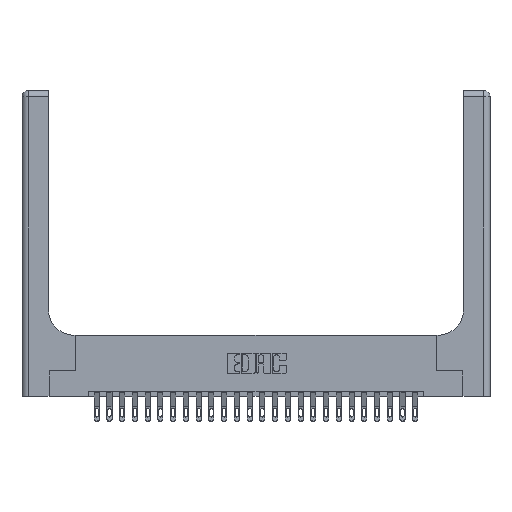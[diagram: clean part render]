
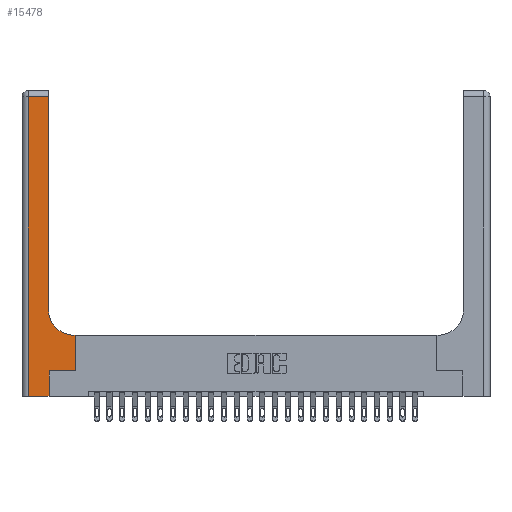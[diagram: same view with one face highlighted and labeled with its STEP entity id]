
A CAD part, top view. The second image highlights one B-rep face of the part: STEP entity #15478.
In plain terms, the highlighted planar face has unit normal (0, 0, 1).
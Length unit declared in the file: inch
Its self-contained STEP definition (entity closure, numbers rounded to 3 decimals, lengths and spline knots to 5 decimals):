
#1014 = CARTESIAN_POINT ( 'NONE',  ( 0.26, 0.85, 0.37 ) ) ;
#1389 = EDGE_CURVE ( 'NONE', #7371, #19761, #3954, .T. ) ;
#1465 = LINE ( 'NONE', #8981, #24023 ) ;
#1598 = ORIENTED_EDGE ( 'NONE', *, *, #18010, .T. ) ;
#1898 = EDGE_CURVE ( 'NONE', #4149, #11383, #24601, .T. ) ;
#1945 = LINE ( 'NONE', #6008, #16752 ) ;
#2330 = DIRECTION ( 'NONE',  ( 0., 1., 0. ) ) ;
#3013 = VECTOR ( 'NONE', #18596, 39.37008 ) ;
#3954 = CIRCLE ( 'NONE', #10452, 0.25 ) ;
#4149 = VERTEX_POINT ( 'NONE', #20204 ) ;
#4366 = DIRECTION ( 'NONE',  ( 0., 1., 0. ) ) ;
#4410 = VERTEX_POINT ( 'NONE', #11803 ) ;
#4549 = EDGE_LOOP ( 'NONE', ( #18722, #13745, #19263, #1598, #19499, #21792, #6718, #7309, #8735 ) ) ;
#5211 = CARTESIAN_POINT ( 'NONE',  ( 0., 2.94, 0.37 ) ) ;
#6008 = CARTESIAN_POINT ( 'NONE',  ( 0., 0., 0.37 ) ) ;
#6191 = DIRECTION ( 'NONE',  ( -1., 0., 0. ) ) ;
#6286 = CARTESIAN_POINT ( 'NONE',  ( 0.265, 0., 0.37 ) ) ;
#6718 = ORIENTED_EDGE ( 'NONE', *, *, #10161, .T. ) ;
#7309 = ORIENTED_EDGE ( 'NONE', *, *, #24909, .T. ) ;
#7371 = VERTEX_POINT ( 'NONE', #11043 ) ;
#7936 = LINE ( 'NONE', #15918, #16631 ) ;
#8138 = CARTESIAN_POINT ( 'NONE',  ( 0.26, 0.6, 0.37 ) ) ;
#8153 = CARTESIAN_POINT ( 'NONE',  ( 0.06, 2.94, 0.37 ) ) ;
#8735 = ORIENTED_EDGE ( 'NONE', *, *, #1389, .T. ) ;
#8981 = CARTESIAN_POINT ( 'NONE',  ( 0.26, 3., 0.37 ) ) ;
#9697 = DIRECTION ( 'NONE',  ( 1., 0., 0. ) ) ;
#9804 = AXIS2_PLACEMENT_3D ( 'NONE', #15721, #9871, #6191 ) ;
#9871 = DIRECTION ( 'NONE',  ( 0., 0., -1. ) ) ;
#10161 = EDGE_CURVE ( 'NONE', #11383, #4410, #7936, .T. ) ;
#10452 = AXIS2_PLACEMENT_3D ( 'NONE', #15229, #15479, #13464 ) ;
#11038 = CARTESIAN_POINT ( 'NONE',  ( 0.06, 0., 0.37 ) ) ;
#11043 = CARTESIAN_POINT ( 'NONE',  ( 0.51, 0.6, 0.37 ) ) ;
#11187 = VECTOR ( 'NONE', #25009, 39.37008 ) ;
#11383 = VERTEX_POINT ( 'NONE', #19030 ) ;
#11803 = CARTESIAN_POINT ( 'NONE',  ( 0.528, 0.6, 0.37 ) ) ;
#12971 = DIRECTION ( 'NONE',  ( -1., 0., 0. ) ) ;
#13177 = CARTESIAN_POINT ( 'NONE',  ( 0.265, 0.25, 0.37 ) ) ;
#13186 = EDGE_CURVE ( 'NONE', #17168, #4149, #23682, .T. ) ;
#13464 = DIRECTION ( 'NONE',  ( 1., 0., 0. ) ) ;
#13709 = LINE ( 'NONE', #21306, #14698 ) ;
#13745 = ORIENTED_EDGE ( 'NONE', *, *, #19863, .T. ) ;
#14698 = VECTOR ( 'NONE', #19912, 39.37008 ) ;
#15229 = CARTESIAN_POINT ( 'NONE',  ( 0.51, 0.85, 0.37 ) ) ;
#15267 = VERTEX_POINT ( 'NONE', #11038 ) ;
#15450 = EDGE_CURVE ( 'NONE', #21460, #15267, #13709, .T. ) ;
#15478 = ADVANCED_FACE ( 'NONE', ( #19655 ), #19789, .F. ) ;
#15479 = DIRECTION ( 'NONE',  ( 0., 0., -1. ) ) ;
#15721 = CARTESIAN_POINT ( 'NONE',  ( 0., 3., 0.37 ) ) ;
#15857 = EDGE_CURVE ( 'NONE', #19761, #17835, #1465, .T. ) ;
#15918 = CARTESIAN_POINT ( 'NONE',  ( 0.528, 0.25, 0.37 ) ) ;
#16631 = VECTOR ( 'NONE', #2330, 39.37008 ) ;
#16752 = VECTOR ( 'NONE', #9697, 39.37008 ) ;
#17168 = VERTEX_POINT ( 'NONE', #20784 ) ;
#17288 = LINE ( 'NONE', #8138, #11187 ) ;
#17835 = VERTEX_POINT ( 'NONE', #22666 ) ;
#18010 = EDGE_CURVE ( 'NONE', #15267, #17168, #1945, .T. ) ;
#18596 = DIRECTION ( 'NONE',  ( 1., 0., 0. ) ) ;
#18722 = ORIENTED_EDGE ( 'NONE', *, *, #15857, .T. ) ;
#19030 = CARTESIAN_POINT ( 'NONE',  ( 0.528, 0.25, 0.37 ) ) ;
#19263 = ORIENTED_EDGE ( 'NONE', *, *, #15450, .T. ) ;
#19499 = ORIENTED_EDGE ( 'NONE', *, *, #13186, .T. ) ;
#19655 = FACE_OUTER_BOUND ( 'NONE', #4549, .T. ) ;
#19761 = VERTEX_POINT ( 'NONE', #1014 ) ;
#19789 = PLANE ( 'NONE',  #9804 ) ;
#19863 = EDGE_CURVE ( 'NONE', #17835, #21460, #22616, .T. ) ;
#19902 = VECTOR ( 'NONE', #4366, 39.37008 ) ;
#19912 = DIRECTION ( 'NONE',  ( 0., -1., 0. ) ) ;
#20048 = VECTOR ( 'NONE', #12971, 39.37008 ) ;
#20204 = CARTESIAN_POINT ( 'NONE',  ( 0.265, 0.25, 0.37 ) ) ;
#20657 = DIRECTION ( 'NONE',  ( 0., 1., 0. ) ) ;
#20784 = CARTESIAN_POINT ( 'NONE',  ( 0.265, 0., 0.37 ) ) ;
#21306 = CARTESIAN_POINT ( 'NONE',  ( 0.06, 3., 0.37 ) ) ;
#21460 = VERTEX_POINT ( 'NONE', #8153 ) ;
#21792 = ORIENTED_EDGE ( 'NONE', *, *, #1898, .T. ) ;
#22616 = LINE ( 'NONE', #5211, #20048 ) ;
#22666 = CARTESIAN_POINT ( 'NONE',  ( 0.26, 2.94, 0.37 ) ) ;
#23682 = LINE ( 'NONE', #6286, #19902 ) ;
#24023 = VECTOR ( 'NONE', #20657, 39.37008 ) ;
#24601 = LINE ( 'NONE', #13177, #3013 ) ;
#24909 = EDGE_CURVE ( 'NONE', #4410, #7371, #17288, .T. ) ;
#25009 = DIRECTION ( 'NONE',  ( -1., 0., 0. ) ) ;
